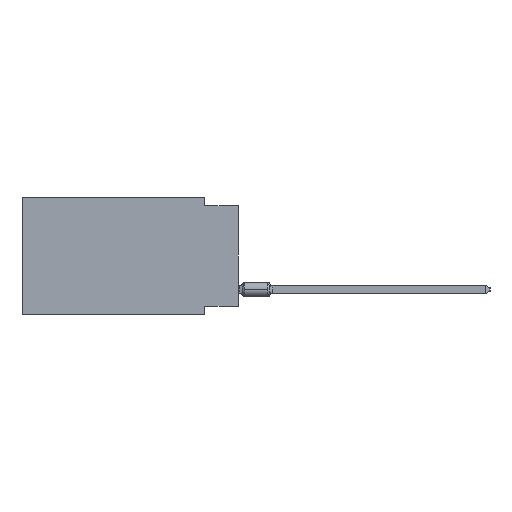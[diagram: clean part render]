
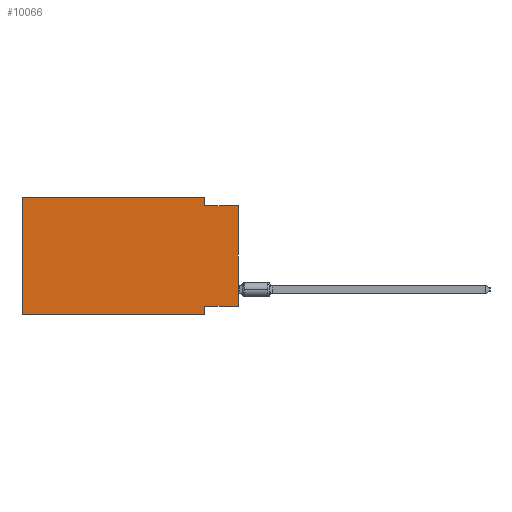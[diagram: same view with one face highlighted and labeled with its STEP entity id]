
A CAD part, left-side view. The second image highlights one B-rep face of the part: STEP entity #10066.
In plain terms, the highlighted planar face has unit normal (-1, 0, 0).
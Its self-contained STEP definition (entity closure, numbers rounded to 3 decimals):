
#1732 = ORIENTED_EDGE ( 'NONE', *, *, #24908, .F. ) ;
#1877 = FACE_OUTER_BOUND ( 'NONE', #5878, .T. ) ;
#2788 = LINE ( 'NONE', #30992, #18384 ) ;
#3768 = VERTEX_POINT ( 'NONE', #27512 ) ;
#4409 = VECTOR ( 'NONE', #4459, 1000. ) ;
#4459 = DIRECTION ( 'NONE',  ( 0., -1., 0. ) ) ;
#5712 = VERTEX_POINT ( 'NONE', #34173 ) ;
#5878 = EDGE_LOOP ( 'NONE', ( #51661, #42183, #46561, #31558, #19968, #32903, #20177, #1732 ) ) ;
#6196 = VECTOR ( 'NONE', #18565, 1000. ) ;
#6361 = LINE ( 'NONE', #46149, #23860 ) ;
#7084 = CARTESIAN_POINT ( 'NONE',  ( 0., 2.54, -8.89 ) ) ;
#7499 = VERTEX_POINT ( 'NONE', #18293 ) ;
#9261 = DIRECTION ( 'NONE',  ( 0., 0., -1. ) ) ;
#10066 = ADVANCED_FACE ( 'NONE', ( #1877 ), #45396, .F. ) ;
#10090 = CARTESIAN_POINT ( 'NONE',  ( 0., 16.383, 0. ) ) ;
#10431 = CARTESIAN_POINT ( 'NONE',  ( 0., 2.54, -8.89 ) ) ;
#10458 = DIRECTION ( 'NONE',  ( 0., 0., 1. ) ) ;
#10876 = CARTESIAN_POINT ( 'NONE',  ( 0., 0., -8.255 ) ) ;
#12664 = VERTEX_POINT ( 'NONE', #35314 ) ;
#14408 = EDGE_CURVE ( 'NONE', #3768, #32072, #2788, .T. ) ;
#16823 = CARTESIAN_POINT ( 'NONE',  ( 0., 16.383, -8.89 ) ) ;
#17166 = VECTOR ( 'NONE', #39368, 1000. ) ;
#18040 = CARTESIAN_POINT ( 'NONE',  ( 0., 2.54, -8.255 ) ) ;
#18293 = CARTESIAN_POINT ( 'NONE',  ( 0., 0., -0.635 ) ) ;
#18384 = VECTOR ( 'NONE', #10458, 1000. ) ;
#18565 = DIRECTION ( 'NONE',  ( 0., 0., -1. ) ) ;
#18989 = CARTESIAN_POINT ( 'NONE',  ( 0., 16.383, 0. ) ) ;
#19012 = EDGE_CURVE ( 'NONE', #26641, #12664, #32438, .T. ) ;
#19968 = ORIENTED_EDGE ( 'NONE', *, *, #14408, .F. ) ;
#20177 = ORIENTED_EDGE ( 'NONE', *, *, #49963, .F. ) ;
#20387 = LINE ( 'NONE', #44929, #49851 ) ;
#20917 = EDGE_CURVE ( 'NONE', #5712, #7499, #20387, .T. ) ;
#23860 = VECTOR ( 'NONE', #37491, 1000. ) ;
#23914 = AXIS2_PLACEMENT_3D ( 'NONE', #45931, #33526, #9261 ) ;
#24134 = VERTEX_POINT ( 'NONE', #18040 ) ;
#24908 = EDGE_CURVE ( 'NONE', #5712, #24134, #48052, .T. ) ;
#26641 = VERTEX_POINT ( 'NONE', #43408 ) ;
#27512 = CARTESIAN_POINT ( 'NONE',  ( 0., 16.383, -8.89 ) ) ;
#29002 = LINE ( 'NONE', #16823, #4409 ) ;
#30607 = LINE ( 'NONE', #18989, #43911 ) ;
#30992 = CARTESIAN_POINT ( 'NONE',  ( 0., 16.383, 0. ) ) ;
#31558 = ORIENTED_EDGE ( 'NONE', *, *, #36094, .F. ) ;
#31639 = VERTEX_POINT ( 'NONE', #7084 ) ;
#32072 = VERTEX_POINT ( 'NONE', #10090 ) ;
#32438 = LINE ( 'NONE', #44536, #37926 ) ;
#32903 = ORIENTED_EDGE ( 'NONE', *, *, #41200, .T. ) ;
#33526 = DIRECTION ( 'NONE',  ( 1., 0., 0. ) ) ;
#34173 = CARTESIAN_POINT ( 'NONE',  ( 0., 0., -8.255 ) ) ;
#35314 = CARTESIAN_POINT ( 'NONE',  ( 0., 2.54, -0.635 ) ) ;
#35491 = DIRECTION ( 'NONE',  ( 0., 0., 1. ) ) ;
#36094 = EDGE_CURVE ( 'NONE', #32072, #26641, #30607, .T. ) ;
#37491 = DIRECTION ( 'NONE',  ( 0., -1., 0. ) ) ;
#37554 = DIRECTION ( 'NONE',  ( 0., -1., 0. ) ) ;
#37926 = VECTOR ( 'NONE', #44299, 1000. ) ;
#38531 = EDGE_CURVE ( 'NONE', #12664, #7499, #6361, .T. ) ;
#39368 = DIRECTION ( 'NONE',  ( 0., 1., 0. ) ) ;
#41200 = EDGE_CURVE ( 'NONE', #3768, #31639, #29002, .T. ) ;
#42183 = ORIENTED_EDGE ( 'NONE', *, *, #38531, .F. ) ;
#43408 = CARTESIAN_POINT ( 'NONE',  ( 0., 2.54, 0. ) ) ;
#43911 = VECTOR ( 'NONE', #37554, 1000. ) ;
#44299 = DIRECTION ( 'NONE',  ( 0., 0., -1. ) ) ;
#44536 = CARTESIAN_POINT ( 'NONE',  ( 0., 2.54, 0. ) ) ;
#44929 = CARTESIAN_POINT ( 'NONE',  ( 0., 0., 0. ) ) ;
#45396 = PLANE ( 'NONE',  #23914 ) ;
#45931 = CARTESIAN_POINT ( 'NONE',  ( 0., 16.383, 0. ) ) ;
#46149 = CARTESIAN_POINT ( 'NONE',  ( 0., 0., -0.635 ) ) ;
#46561 = ORIENTED_EDGE ( 'NONE', *, *, #19012, .F. ) ;
#48052 = LINE ( 'NONE', #10876, #17166 ) ;
#49851 = VECTOR ( 'NONE', #35491, 1000. ) ;
#49963 = EDGE_CURVE ( 'NONE', #24134, #31639, #51520, .T. ) ;
#51520 = LINE ( 'NONE', #10431, #6196 ) ;
#51661 = ORIENTED_EDGE ( 'NONE', *, *, #20917, .T. ) ;
